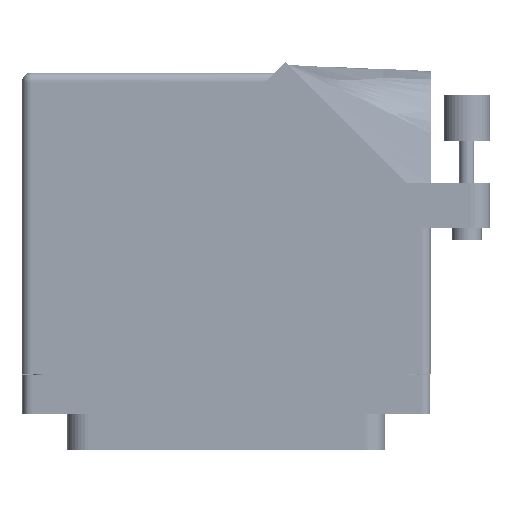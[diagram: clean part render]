
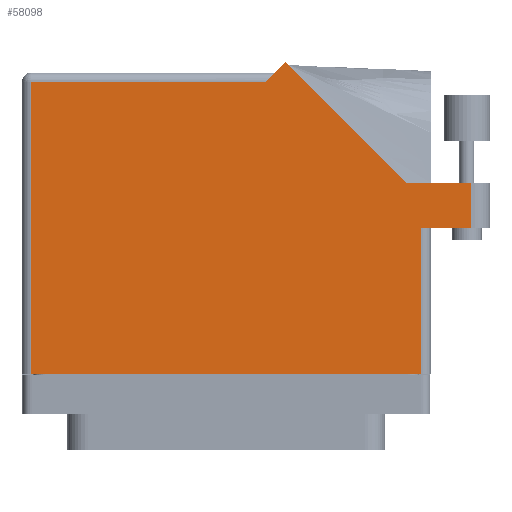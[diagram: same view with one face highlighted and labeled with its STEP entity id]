
A CAD part, front view. The second image highlights one B-rep face of the part: STEP entity #58098.
In plain terms, the highlighted face is planar.
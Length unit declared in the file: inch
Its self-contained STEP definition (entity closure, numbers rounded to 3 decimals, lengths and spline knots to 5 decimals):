
#883 = CARTESIAN_POINT ( 'NONE',  ( -1.3155, -0.1, 0.765 ) ) ;
#1386 = DIRECTION ( 'NONE',  ( -0.707, 0.707, 0. ) ) ;
#2543 = VECTOR ( 'NONE', #16487, 39.37008 ) ;
#2689 = CARTESIAN_POINT ( 'NONE',  ( -1.3155, 1.868, 0.765 ) ) ;
#4185 = FACE_OUTER_BOUND ( 'NONE', #8211, .T. ) ;
#4891 = CARTESIAN_POINT ( 'NONE',  ( 1.6525, 1.187, 0.765 ) ) ;
#5860 = VERTEX_POINT ( 'NONE', #883 ) ;
#6522 = CARTESIAN_POINT ( 'NONE',  ( 1.3155, 0.88, 0.765 ) ) ;
#6971 = VERTEX_POINT ( 'NONE', #82386 ) ;
#7254 = ORIENTED_EDGE ( 'NONE', *, *, #48934, .T. ) ;
#8211 = EDGE_LOOP ( 'NONE', ( #7254, #70908, #36367, #82434, #42381, #35255, #58927, #32480, #68584 ) ) ;
#8571 = CARTESIAN_POINT ( 'NONE',  ( 1.3155, 0.88, 0.765 ) ) ;
#12153 = VERTEX_POINT ( 'NONE', #47997 ) ;
#16174 = CARTESIAN_POINT ( 'NONE',  ( 1.3775, 0.88, 0.765 ) ) ;
#16487 = DIRECTION ( 'NONE',  ( -0.707, -0.707, 0. ) ) ;
#18006 = VECTOR ( 'NONE', #64389, 39.37008 ) ;
#19830 = DIRECTION ( 'NONE',  ( -1., 0., 0. ) ) ;
#21063 = VECTOR ( 'NONE', #1386, 39.37008 ) ;
#25762 = VECTOR ( 'NONE', #19830, 39.37008 ) ;
#26219 = LINE ( 'NONE', #56547, #2543 ) ;
#28792 = VECTOR ( 'NONE', #62897, 39.37008 ) ;
#29422 = DIRECTION ( 'NONE',  ( 0., 1., 0. ) ) ;
#32480 = ORIENTED_EDGE ( 'NONE', *, *, #36768, .T. ) ;
#33050 = EDGE_CURVE ( 'NONE', #82334, #12153, #26219, .T. ) ;
#33278 = PLANE ( 'NONE',  #65093 ) ;
#34623 = VERTEX_POINT ( 'NONE', #35223 ) ;
#35103 = LINE ( 'NONE', #8571, #58848 ) ;
#35223 = CARTESIAN_POINT ( 'NONE',  ( 1.6525, 0.88, 0.765 ) ) ;
#35255 = ORIENTED_EDGE ( 'NONE', *, *, #81912, .T. ) ;
#36367 = ORIENTED_EDGE ( 'NONE', *, *, #63650, .T. ) ;
#36768 = EDGE_CURVE ( 'NONE', #5860, #6971, #59046, .T. ) ;
#40682 = CARTESIAN_POINT ( 'NONE',  ( -1.3775, 1.868, 0.765 ) ) ;
#42381 = ORIENTED_EDGE ( 'NONE', *, *, #33050, .T. ) ;
#43968 = VECTOR ( 'NONE', #45861, 39.37008 ) ;
#45830 = DIRECTION ( 'NONE',  ( 0., -1., 0. ) ) ;
#45861 = DIRECTION ( 'NONE',  ( 1., 0., 0. ) ) ;
#46179 = EDGE_CURVE ( 'NONE', #34623, #87353, #47508, .T. ) ;
#46862 = CARTESIAN_POINT ( 'NONE',  ( -1.3775, 1.93, 0.765 ) ) ;
#47508 = LINE ( 'NONE', #72146, #56079 ) ;
#47997 = CARTESIAN_POINT ( 'NONE',  ( 0.2655, 1.868, 0.765 ) ) ;
#48934 = EDGE_CURVE ( 'NONE', #79075, #34623, #58982, .T. ) ;
#53125 = DIRECTION ( 'NONE',  ( 0., 0., -1. ) ) ;
#54407 = CARTESIAN_POINT ( 'NONE',  ( 1.7775, 1.187, 0.765 ) ) ;
#56079 = VECTOR ( 'NONE', #59426, 39.37008 ) ;
#56547 = CARTESIAN_POINT ( 'NONE',  ( 0.3275, 1.93, 0.765 ) ) ;
#57266 = VERTEX_POINT ( 'NONE', #2689 ) ;
#57900 = DIRECTION ( 'NONE',  ( -1., 0., 0. ) ) ;
#58098 = ADVANCED_FACE ( 'NONE', ( #4185 ), #33278, .F. ) ;
#58848 = VECTOR ( 'NONE', #29422, 39.37008 ) ;
#58927 = ORIENTED_EDGE ( 'NONE', *, *, #80176, .T. ) ;
#58982 = LINE ( 'NONE', #16174, #18006 ) ;
#59046 = LINE ( 'NONE', #59977, #43968 ) ;
#59426 = DIRECTION ( 'NONE',  ( 0., 1., 0. ) ) ;
#59977 = CARTESIAN_POINT ( 'NONE',  ( -1.3775, -0.1, 0.765 ) ) ;
#60548 = CARTESIAN_POINT ( 'NONE',  ( -1.3155, -0.1, 0.765 ) ) ;
#62455 = LINE ( 'NONE', #40682, #25762 ) ;
#62897 = DIRECTION ( 'NONE',  ( -1., 0., 0. ) ) ;
#63103 = CARTESIAN_POINT ( 'NONE',  ( 0.39821, 2.00071, 0.765 ) ) ;
#63650 = EDGE_CURVE ( 'NONE', #87353, #81032, #78501, .T. ) ;
#63914 = VECTOR ( 'NONE', #45830, 39.37008 ) ;
#64236 = LINE ( 'NONE', #84588, #21063 ) ;
#64362 = EDGE_CURVE ( 'NONE', #81032, #82334, #64236, .T. ) ;
#64388 = EDGE_CURVE ( 'NONE', #6971, #79075, #35103, .T. ) ;
#64389 = DIRECTION ( 'NONE',  ( 1., 0., 0. ) ) ;
#65093 = AXIS2_PLACEMENT_3D ( 'NONE', #46862, #53125, #57900 ) ;
#68584 = ORIENTED_EDGE ( 'NONE', *, *, #64388, .T. ) ;
#70908 = ORIENTED_EDGE ( 'NONE', *, *, #46179, .T. ) ;
#72146 = CARTESIAN_POINT ( 'NONE',  ( 1.6525, 1.187, 0.765 ) ) ;
#75329 = CARTESIAN_POINT ( 'NONE',  ( 1.21192, 1.187, 0.765 ) ) ;
#78004 = LINE ( 'NONE', #60548, #63914 ) ;
#78501 = LINE ( 'NONE', #54407, #28792 ) ;
#79075 = VERTEX_POINT ( 'NONE', #6522 ) ;
#80176 = EDGE_CURVE ( 'NONE', #57266, #5860, #78004, .T. ) ;
#81032 = VERTEX_POINT ( 'NONE', #75329 ) ;
#81912 = EDGE_CURVE ( 'NONE', #12153, #57266, #62455, .T. ) ;
#82334 = VERTEX_POINT ( 'NONE', #63103 ) ;
#82386 = CARTESIAN_POINT ( 'NONE',  ( 1.3155, -0.1, 0.765 ) ) ;
#82434 = ORIENTED_EDGE ( 'NONE', *, *, #64362, .T. ) ;
#84588 = CARTESIAN_POINT ( 'NONE',  ( 1.21192, 1.187, 0.765 ) ) ;
#87353 = VERTEX_POINT ( 'NONE', #4891 ) ;
